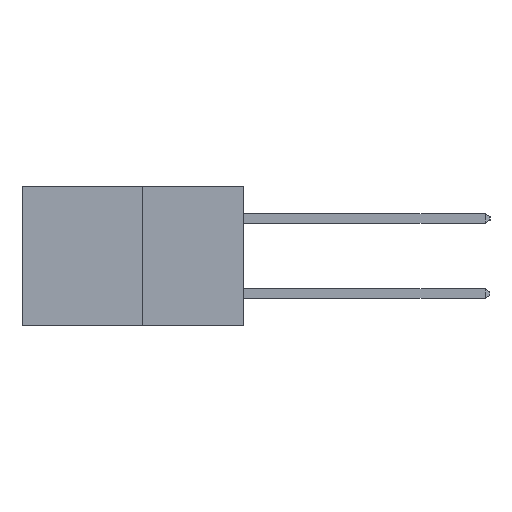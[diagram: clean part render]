
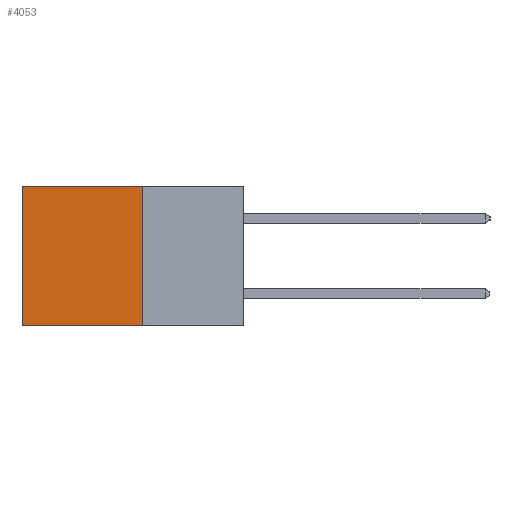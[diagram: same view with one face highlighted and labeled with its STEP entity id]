
A CAD part, left-side view. The second image highlights one B-rep face of the part: STEP entity #4053.
In plain terms, the highlighted planar face has unit normal (-1, 0, 0).
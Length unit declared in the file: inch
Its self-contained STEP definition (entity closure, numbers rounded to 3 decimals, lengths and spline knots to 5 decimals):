
#432 = LINE ( 'NONE', #7094, #4672 ) ;
#628 = LINE ( 'NONE', #4983, #7060 ) ;
#1106 = PLANE ( 'NONE',  #3393 ) ;
#1111 = CARTESIAN_POINT ( 'NONE',  ( 0.277, 0.27, -0.37 ) ) ;
#1613 = ORIENTED_EDGE ( 'NONE', *, *, #7363, .F. ) ;
#1853 = CARTESIAN_POINT ( 'NONE',  ( 0.277, 0.27, -0.37 ) ) ;
#1857 = CARTESIAN_POINT ( 'NONE',  ( 0.277, 0.59, 0. ) ) ;
#2220 = FACE_OUTER_BOUND ( 'NONE', #5545, .T. ) ;
#2238 = EDGE_CURVE ( 'NONE', #7907, #9575, #4242, .T. ) ;
#2967 = ORIENTED_EDGE ( 'NONE', *, *, #8943, .F. ) ;
#3143 = ORIENTED_EDGE ( 'NONE', *, *, #2238, .T. ) ;
#3393 = AXIS2_PLACEMENT_3D ( 'NONE', #1853, #8121, #10452 ) ;
#4053 = ADVANCED_FACE ( 'NONE', ( #2220 ), #1106, .F. ) ;
#4242 = LINE ( 'NONE', #6266, #5868 ) ;
#4516 = EDGE_CURVE ( 'NONE', #9575, #7945, #432, .T. ) ;
#4672 = VECTOR ( 'NONE', #7018, 39.37008 ) ;
#4983 = CARTESIAN_POINT ( 'NONE',  ( 0.277, 0.27, -0.37 ) ) ;
#5075 = DIRECTION ( 'NONE',  ( 0., 0., -1. ) ) ;
#5354 = ORIENTED_EDGE ( 'NONE', *, *, #4516, .T. ) ;
#5545 = EDGE_LOOP ( 'NONE', ( #5354, #2967, #1613, #3143 ) ) ;
#5736 = DIRECTION ( 'NONE',  ( 0., 1., 0. ) ) ;
#5868 = VECTOR ( 'NONE', #6190, 39.37008 ) ;
#5983 = CARTESIAN_POINT ( 'NONE',  ( 0.277, 0.27, -0.37 ) ) ;
#6190 = DIRECTION ( 'NONE',  ( 0., 1., 0. ) ) ;
#6266 = CARTESIAN_POINT ( 'NONE',  ( 0.277, 0.27, 0. ) ) ;
#6283 = CARTESIAN_POINT ( 'NONE',  ( 0.277, 0.59, -0.37 ) ) ;
#6798 = LINE ( 'NONE', #5983, #8749 ) ;
#7018 = DIRECTION ( 'NONE',  ( 0., 0., -1. ) ) ;
#7060 = VECTOR ( 'NONE', #5075, 39.37008 ) ;
#7094 = CARTESIAN_POINT ( 'NONE',  ( 0.277, 0.59, -0.37 ) ) ;
#7363 = EDGE_CURVE ( 'NONE', #7907, #8327, #628, .T. ) ;
#7593 = CARTESIAN_POINT ( 'NONE',  ( 0.277, 0.27, 0. ) ) ;
#7907 = VERTEX_POINT ( 'NONE', #7593 ) ;
#7945 = VERTEX_POINT ( 'NONE', #6283 ) ;
#8121 = DIRECTION ( 'NONE',  ( 1., 0., 0. ) ) ;
#8327 = VERTEX_POINT ( 'NONE', #1111 ) ;
#8749 = VECTOR ( 'NONE', #5736, 39.37008 ) ;
#8943 = EDGE_CURVE ( 'NONE', #8327, #7945, #6798, .T. ) ;
#9575 = VERTEX_POINT ( 'NONE', #1857 ) ;
#10452 = DIRECTION ( 'NONE',  ( 0., 0., -1. ) ) ;
